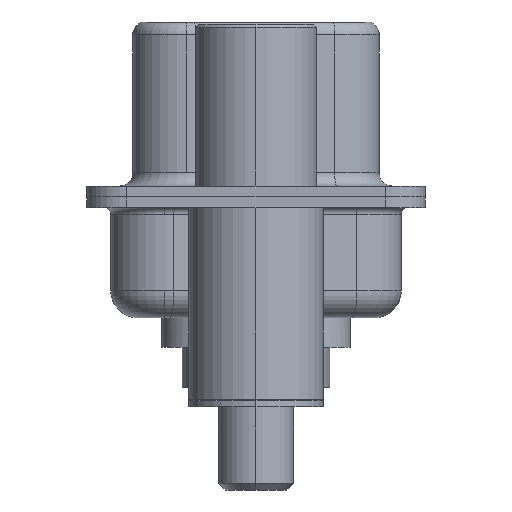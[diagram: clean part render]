
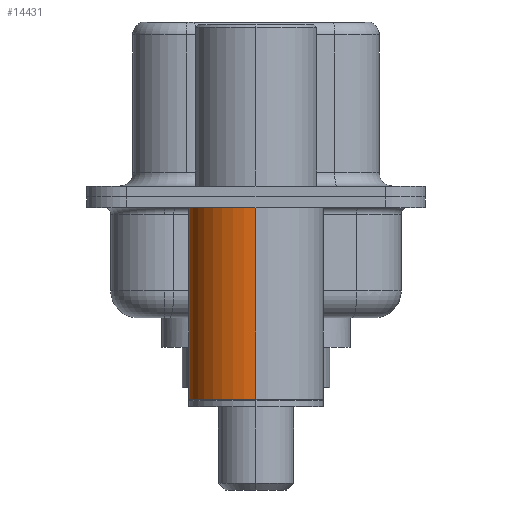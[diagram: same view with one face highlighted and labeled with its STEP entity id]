
A CAD part, left-side view. The second image highlights one B-rep face of the part: STEP entity #14431.
In plain terms, the highlighted cylindrical face has radius 2.5 mm (diameter 5 mm), a partial arc.
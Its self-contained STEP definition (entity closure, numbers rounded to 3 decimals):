
#269 = DIRECTION ( 'NONE',  ( 0., 0., 1. ) ) ;
#490 = VERTEX_POINT ( 'NONE', #7147 ) ;
#602 = VERTEX_POINT ( 'NONE', #3099 ) ;
#1042 = CIRCLE ( 'NONE', #7914, 2.5 ) ;
#1172 = DIRECTION ( 'NONE',  ( 0., 0., 1. ) ) ;
#1575 = DIRECTION ( 'NONE',  ( 1., 0., 0. ) ) ;
#1862 = VECTOR ( 'NONE', #8377, 1000. ) ;
#2799 = VECTOR ( 'NONE', #269, 1000. ) ;
#3099 = CARTESIAN_POINT ( 'NONE',  ( -2.5, 0., -0.4 ) ) ;
#4406 = EDGE_CURVE ( 'NONE', #490, #602, #14839, .T. ) ;
#4640 = ORIENTED_EDGE ( 'NONE', *, *, #4406, .T. ) ;
#4989 = DIRECTION ( 'NONE',  ( 1., 0., 0. ) ) ;
#5312 = ORIENTED_EDGE ( 'NONE', *, *, #5776, .F. ) ;
#5315 = DIRECTION ( 'NONE',  ( 1., 0., 0. ) ) ;
#5678 = EDGE_CURVE ( 'NONE', #8121, #602, #1042, .T. ) ;
#5776 = EDGE_CURVE ( 'NONE', #6062, #8121, #15712, .T. ) ;
#5832 = AXIS2_PLACEMENT_3D ( 'NONE', #13791, #1172, #4989 ) ;
#5871 = EDGE_CURVE ( 'NONE', #6062, #490, #9643, .T. ) ;
#6062 = VERTEX_POINT ( 'NONE', #13209 ) ;
#7147 = CARTESIAN_POINT ( 'NONE',  ( -2.5, 0., -7.525 ) ) ;
#7914 = AXIS2_PLACEMENT_3D ( 'NONE', #15965, #15933, #5315 ) ;
#8121 = VERTEX_POINT ( 'NONE', #10114 ) ;
#8377 = DIRECTION ( 'NONE',  ( 0., 0., 1. ) ) ;
#8836 = EDGE_LOOP ( 'NONE', ( #9566, #4640, #11945, #5312 ) ) ;
#9276 = CARTESIAN_POINT ( 'NONE',  ( 2.5, 0., 0.581 ) ) ;
#9566 = ORIENTED_EDGE ( 'NONE', *, *, #5871, .T. ) ;
#9643 = CIRCLE ( 'NONE', #5832, 2.5 ) ;
#10114 = CARTESIAN_POINT ( 'NONE',  ( 2.5, 0., -0.4 ) ) ;
#10524 = CARTESIAN_POINT ( 'NONE',  ( 0., 0., 0.581 ) ) ;
#11333 = FACE_OUTER_BOUND ( 'NONE', #8836, .T. ) ;
#11763 = DIRECTION ( 'NONE',  ( 0., 0., 1. ) ) ;
#11945 = ORIENTED_EDGE ( 'NONE', *, *, #5678, .F. ) ;
#13209 = CARTESIAN_POINT ( 'NONE',  ( 2.5, 0., -7.525 ) ) ;
#13791 = CARTESIAN_POINT ( 'NONE',  ( 0., 0., -7.525 ) ) ;
#14163 = CYLINDRICAL_SURFACE ( 'NONE', #15918, 2.5 ) ;
#14431 = ADVANCED_FACE ( 'NONE', ( #11333 ), #14163, .T. ) ;
#14839 = LINE ( 'NONE', #15182, #1862 ) ;
#15182 = CARTESIAN_POINT ( 'NONE',  ( -2.5, 0., 0.581 ) ) ;
#15712 = LINE ( 'NONE', #9276, #2799 ) ;
#15918 = AXIS2_PLACEMENT_3D ( 'NONE', #10524, #11763, #1575 ) ;
#15933 = DIRECTION ( 'NONE',  ( 0., 0., 1. ) ) ;
#15965 = CARTESIAN_POINT ( 'NONE',  ( 0., 0., -0.4 ) ) ;
